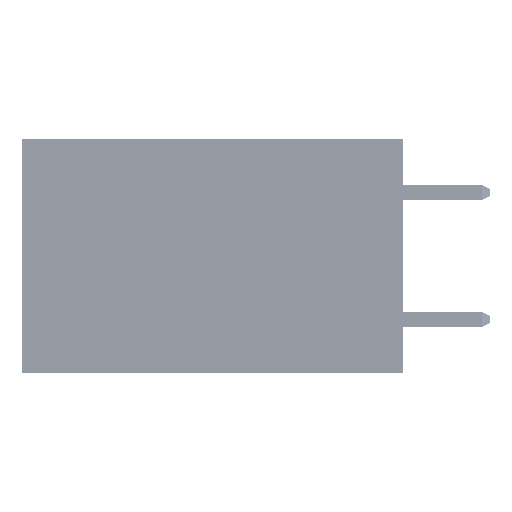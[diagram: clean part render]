
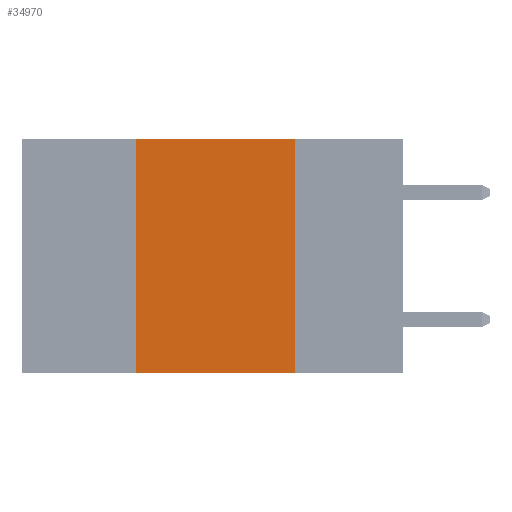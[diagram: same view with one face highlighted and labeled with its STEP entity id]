
A CAD part, left-side view. The second image highlights one B-rep face of the part: STEP entity #34970.
In plain terms, the highlighted planar face has unit normal (-1, 0, 0).
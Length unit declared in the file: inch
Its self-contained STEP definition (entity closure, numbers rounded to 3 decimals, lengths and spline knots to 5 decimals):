
#1120 = EDGE_CURVE ( 'NONE', #48599, #20504, #22179, .T. ) ;
#2132 = VERTEX_POINT ( 'NONE', #35216 ) ;
#2206 = EDGE_CURVE ( 'NONE', #2132, #11339, #43885, .T. ) ;
#3666 = CARTESIAN_POINT ( 'NONE',  ( 0., 0.6, 0. ) ) ;
#4428 = ORIENTED_EDGE ( 'NONE', *, *, #1120, .F. ) ;
#7754 = ORIENTED_EDGE ( 'NONE', *, *, #37674, .T. ) ;
#8332 = VECTOR ( 'NONE', #12023, 39.37008 ) ;
#9568 = VECTOR ( 'NONE', #40329, 39.37008 ) ;
#11339 = VERTEX_POINT ( 'NONE', #38181 ) ;
#11897 = CARTESIAN_POINT ( 'NONE',  ( 0., 0.42, 0. ) ) ;
#12023 = DIRECTION ( 'NONE',  ( 0., -1., 0. ) ) ;
#12462 = CARTESIAN_POINT ( 'NONE',  ( 0., 0.6, 0. ) ) ;
#12737 = CARTESIAN_POINT ( 'NONE',  ( 0., 0.17, 0. ) ) ;
#12813 = DIRECTION ( 'NONE',  ( 0., 0., -1. ) ) ;
#15320 = LINE ( 'NONE', #36221, #8332 ) ;
#16387 = PLANE ( 'NONE',  #44268 ) ;
#16691 = CARTESIAN_POINT ( 'NONE',  ( 0., 0.17, 0. ) ) ;
#20489 = ORIENTED_EDGE ( 'NONE', *, *, #2206, .F. ) ;
#20504 = VERTEX_POINT ( 'NONE', #37127 ) ;
#22179 = LINE ( 'NONE', #12737, #38673 ) ;
#28047 = DIRECTION ( 'NONE',  ( 0., -1., 0. ) ) ;
#31493 = EDGE_LOOP ( 'NONE', ( #4428, #50066, #20489, #7754 ) ) ;
#32017 = LINE ( 'NONE', #3666, #47927 ) ;
#34970 = ADVANCED_FACE ( 'NONE', ( #35996 ), #16387, .F. ) ;
#35216 = CARTESIAN_POINT ( 'NONE',  ( 0., 0.42, -0.37 ) ) ;
#35996 = FACE_OUTER_BOUND ( 'NONE', #31493, .T. ) ;
#36221 = CARTESIAN_POINT ( 'NONE',  ( 0., 0.6, -0.37 ) ) ;
#36487 = EDGE_CURVE ( 'NONE', #11339, #48599, #32017, .T. ) ;
#37127 = CARTESIAN_POINT ( 'NONE',  ( 0., 0.17, -0.37 ) ) ;
#37674 = EDGE_CURVE ( 'NONE', #2132, #20504, #15320, .T. ) ;
#38181 = CARTESIAN_POINT ( 'NONE',  ( 0., 0.42, 0. ) ) ;
#38673 = VECTOR ( 'NONE', #40983, 39.37008 ) ;
#40329 = DIRECTION ( 'NONE',  ( 0., 0., 1. ) ) ;
#40881 = DIRECTION ( 'NONE',  ( 1., 0., 0. ) ) ;
#40983 = DIRECTION ( 'NONE',  ( 0., 0., -1. ) ) ;
#43885 = LINE ( 'NONE', #11897, #9568 ) ;
#44268 = AXIS2_PLACEMENT_3D ( 'NONE', #12462, #40881, #12813 ) ;
#47927 = VECTOR ( 'NONE', #28047, 39.37008 ) ;
#48599 = VERTEX_POINT ( 'NONE', #16691 ) ;
#50066 = ORIENTED_EDGE ( 'NONE', *, *, #36487, .F. ) ;
